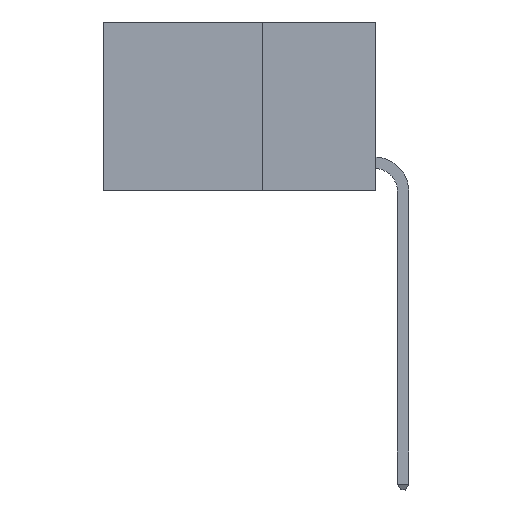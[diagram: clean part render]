
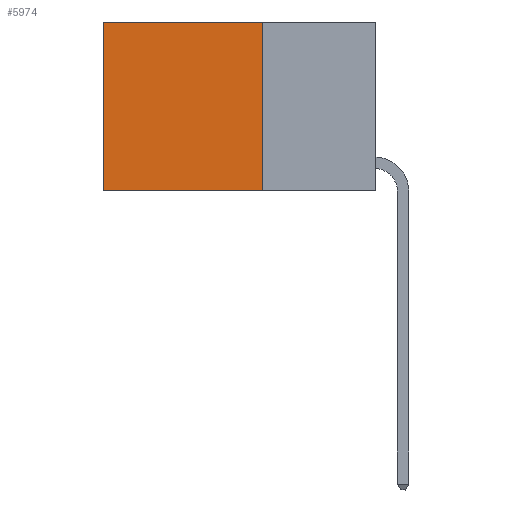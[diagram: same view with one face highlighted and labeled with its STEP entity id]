
A CAD part, left-side view. The second image highlights one B-rep face of the part: STEP entity #5974.
In plain terms, the highlighted planar face has unit normal (-1, 0, 0).
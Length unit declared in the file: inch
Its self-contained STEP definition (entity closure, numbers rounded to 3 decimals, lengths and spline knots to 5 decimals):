
#87 = EDGE_CURVE ( 'NONE', #7169, #17819, #5671, .T. ) ;
#129 = FACE_OUTER_BOUND ( 'NONE', #4864, .T. ) ;
#229 = EDGE_CURVE ( 'NONE', #7169, #4939, #17776, .T. ) ;
#1448 = EDGE_CURVE ( 'NONE', #17819, #4828, #9003, .T. ) ;
#2625 = CARTESIAN_POINT ( 'NONE',  ( 0.2625, 0.25, -0.37 ) ) ;
#3069 = DIRECTION ( 'NONE',  ( 0., 0., -1. ) ) ;
#3519 = CARTESIAN_POINT ( 'NONE',  ( 0.2625, 0.25, -0.37 ) ) ;
#3534 = AXIS2_PLACEMENT_3D ( 'NONE', #8264, #5438, #15538 ) ;
#3535 = DIRECTION ( 'NONE',  ( 0., 0., -1. ) ) ;
#3623 = CARTESIAN_POINT ( 'NONE',  ( 0.2625, 0.6, 0. ) ) ;
#4255 = CARTESIAN_POINT ( 'NONE',  ( 0.2625, 0.25, 0. ) ) ;
#4274 = CARTESIAN_POINT ( 'NONE',  ( 0.2625, 0.6, -0.37 ) ) ;
#4828 = VERTEX_POINT ( 'NONE', #4274 ) ;
#4864 = EDGE_LOOP ( 'NONE', ( #13474, #15128, #17844, #15132 ) ) ;
#4939 = VERTEX_POINT ( 'NONE', #3519 ) ;
#5222 = VECTOR ( 'NONE', #9166, 39.37008 ) ;
#5438 = DIRECTION ( 'NONE',  ( 1., 0., 0. ) ) ;
#5671 = LINE ( 'NONE', #9288, #5222 ) ;
#5974 = ADVANCED_FACE ( 'NONE', ( #129 ), #18258, .F. ) ;
#7169 = VERTEX_POINT ( 'NONE', #15499 ) ;
#8264 = CARTESIAN_POINT ( 'NONE',  ( 0.2625, 0.25, 0. ) ) ;
#9003 = LINE ( 'NONE', #3623, #12844 ) ;
#9166 = DIRECTION ( 'NONE',  ( 0., 1., 0. ) ) ;
#9288 = CARTESIAN_POINT ( 'NONE',  ( 0.2625, 0.25, 0. ) ) ;
#12371 = LINE ( 'NONE', #2625, #15755 ) ;
#12844 = VECTOR ( 'NONE', #3535, 39.37008 ) ;
#13474 = ORIENTED_EDGE ( 'NONE', *, *, #1448, .T. ) ;
#14025 = VECTOR ( 'NONE', #3069, 39.37008 ) ;
#14241 = DIRECTION ( 'NONE',  ( 0., 1., 0. ) ) ;
#15128 = ORIENTED_EDGE ( 'NONE', *, *, #17133, .F. ) ;
#15132 = ORIENTED_EDGE ( 'NONE', *, *, #87, .T. ) ;
#15499 = CARTESIAN_POINT ( 'NONE',  ( 0.2625, 0.25, 0. ) ) ;
#15538 = DIRECTION ( 'NONE',  ( 0., 0., -1. ) ) ;
#15755 = VECTOR ( 'NONE', #14241, 39.37008 ) ;
#17133 = EDGE_CURVE ( 'NONE', #4939, #4828, #12371, .T. ) ;
#17173 = CARTESIAN_POINT ( 'NONE',  ( 0.2625, 0.6, 0. ) ) ;
#17776 = LINE ( 'NONE', #4255, #14025 ) ;
#17819 = VERTEX_POINT ( 'NONE', #17173 ) ;
#17844 = ORIENTED_EDGE ( 'NONE', *, *, #229, .F. ) ;
#18258 = PLANE ( 'NONE',  #3534 ) ;
